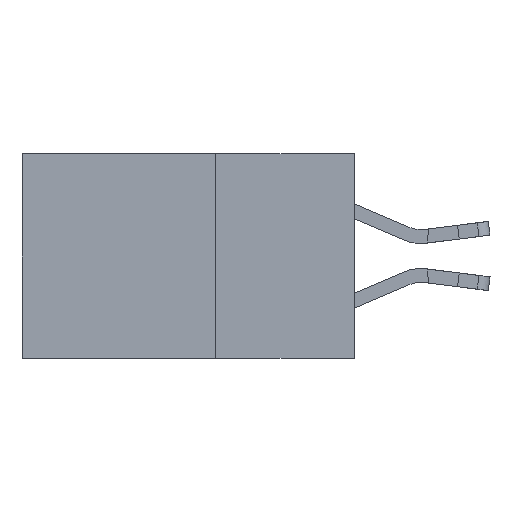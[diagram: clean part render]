
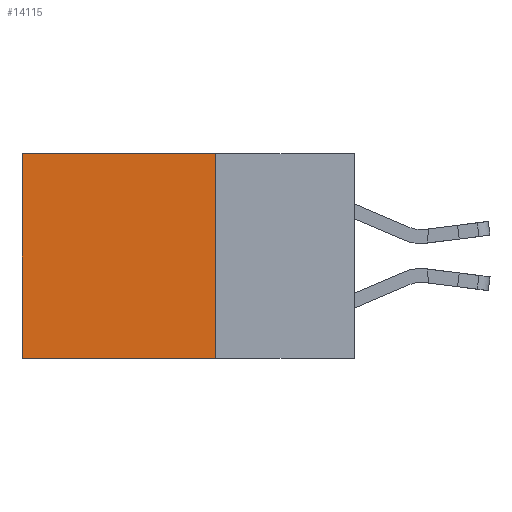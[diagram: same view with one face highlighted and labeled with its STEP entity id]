
A CAD part, left-side view. The second image highlights one B-rep face of the part: STEP entity #14115.
In plain terms, the highlighted planar face has unit normal (-1, 0, 0).
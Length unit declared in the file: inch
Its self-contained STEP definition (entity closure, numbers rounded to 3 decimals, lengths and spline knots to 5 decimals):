
#1056 = CARTESIAN_POINT ( 'NONE',  ( 0.2615, 0.25, -0.37 ) ) ;
#1622 = FACE_OUTER_BOUND ( 'NONE', #16166, .T. ) ;
#1841 = VECTOR ( 'NONE', #2547, 39.37008 ) ;
#2089 = DIRECTION ( 'NONE',  ( 0., 0., -1. ) ) ;
#2298 = CARTESIAN_POINT ( 'NONE',  ( 0.2615, 0.25, 0. ) ) ;
#2395 = VERTEX_POINT ( 'NONE', #8717 ) ;
#2437 = ORIENTED_EDGE ( 'NONE', *, *, #13121, .F. ) ;
#2547 = DIRECTION ( 'NONE',  ( 0., 1., 0. ) ) ;
#2567 = DIRECTION ( 'NONE',  ( 1., 0., 0. ) ) ;
#2647 = DIRECTION ( 'NONE',  ( 0., 0., -1. ) ) ;
#3562 = ORIENTED_EDGE ( 'NONE', *, *, #12372, .T. ) ;
#4026 = VERTEX_POINT ( 'NONE', #2298 ) ;
#5208 = ORIENTED_EDGE ( 'NONE', *, *, #14782, .T. ) ;
#5538 = CARTESIAN_POINT ( 'NONE',  ( 0.2615, 0.6, -0.37 ) ) ;
#6111 = AXIS2_PLACEMENT_3D ( 'NONE', #11835, #2567, #13333 ) ;
#6703 = CARTESIAN_POINT ( 'NONE',  ( 0.2615, 0.25, -0.37 ) ) ;
#7167 = PLANE ( 'NONE',  #6111 ) ;
#7478 = LINE ( 'NONE', #1056, #12070 ) ;
#8717 = CARTESIAN_POINT ( 'NONE',  ( 0.2615, 0.6, 0. ) ) ;
#8948 = VERTEX_POINT ( 'NONE', #5538 ) ;
#10038 = ORIENTED_EDGE ( 'NONE', *, *, #12143, .F. ) ;
#10282 = CARTESIAN_POINT ( 'NONE',  ( 0.2615, 0.25, 0. ) ) ;
#11835 = CARTESIAN_POINT ( 'NONE',  ( 0.2615, 0.25, -0.37 ) ) ;
#11928 = DIRECTION ( 'NONE',  ( 0., 1., 0. ) ) ;
#12070 = VECTOR ( 'NONE', #11928, 39.37008 ) ;
#12143 = EDGE_CURVE ( 'NONE', #4026, #19790, #17941, .T. ) ;
#12372 = EDGE_CURVE ( 'NONE', #2395, #8948, #13267, .T. ) ;
#13121 = EDGE_CURVE ( 'NONE', #19790, #8948, #7478, .T. ) ;
#13267 = LINE ( 'NONE', #14910, #17240 ) ;
#13333 = DIRECTION ( 'NONE',  ( 0., 0., -1. ) ) ;
#14115 = ADVANCED_FACE ( 'NONE', ( #1622 ), #7167, .F. ) ;
#14782 = EDGE_CURVE ( 'NONE', #4026, #2395, #18095, .T. ) ;
#14910 = CARTESIAN_POINT ( 'NONE',  ( 0.2615, 0.6, -0.37 ) ) ;
#16166 = EDGE_LOOP ( 'NONE', ( #3562, #2437, #10038, #5208 ) ) ;
#16705 = CARTESIAN_POINT ( 'NONE',  ( 0.2615, 0.25, -0.37 ) ) ;
#17240 = VECTOR ( 'NONE', #2647, 39.37008 ) ;
#17941 = LINE ( 'NONE', #6703, #18876 ) ;
#18095 = LINE ( 'NONE', #10282, #1841 ) ;
#18876 = VECTOR ( 'NONE', #2089, 39.37008 ) ;
#19790 = VERTEX_POINT ( 'NONE', #16705 ) ;
